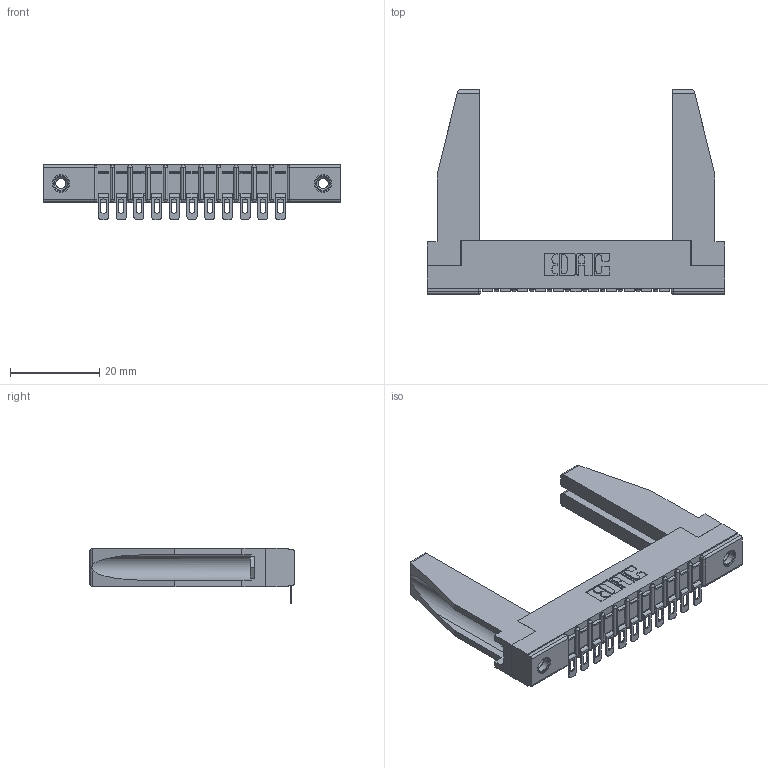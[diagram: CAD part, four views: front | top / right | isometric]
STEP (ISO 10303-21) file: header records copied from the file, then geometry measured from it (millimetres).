
FILE_DESCRIPTION (( 'STEP AP203' ), '1' );
FILE_NAME ('357-011-554-178.STEP', '2019-09-16T19:00:18', ( '' ), ( '' ), 'SwSTEP 2.0', 'SolidWorks 2016', '' );
FILE_SCHEMA (( 'CONFIG_CONTROL_DESIGN' ));
Length unit declared in the file: inch
Products named in the file (5): 307-220-078; 307-290-002_554; 345-250-001_345-250-001-102; 307 Part_.156 Dia Mounting Holes; 357-011-554-178
Assembly tree (16 placements, depth 2):
  357-011-554-178
    307 Part_.156 Dia Mounting Holes
    307-290-002_554  x11
    307-220-078  x2
    345-250-001_345-250-001-102  x2
Bounding box: 66.6 x 45.72 x 12.52 mm (x, y, z)
Volume: 8388.3 mm3; surface area: 11248 mm2
Topology: 16 solids, 16 shells, 1151 faces, 3436 edges, 2248 vertices
Faces by surface type: plane 660, cylinder 451, sphere 24, cone 12, torus 4
Entity records: 16656 total; most frequent: CARTESIAN_POINT 2804, ORIENTED_EDGE 2750, DIRECTION 2701, EDGE_CURVE 1375, VECTOR 1035, LINE 1035, VERTEX_POINT 894, AXIS2_PLACEMENT_3D 833
